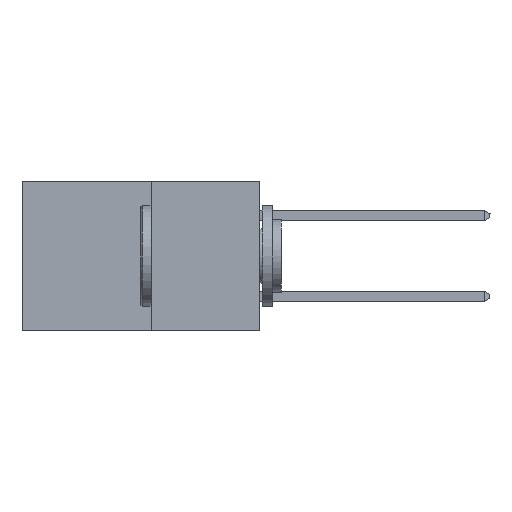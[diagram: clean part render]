
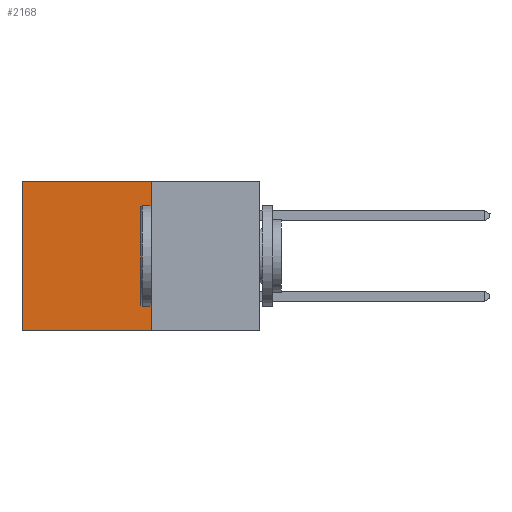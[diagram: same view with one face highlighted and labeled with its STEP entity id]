
A CAD part, left-side view. The second image highlights one B-rep face of the part: STEP entity #2168.
In plain terms, the highlighted planar face has unit normal (-1, 0, 0).
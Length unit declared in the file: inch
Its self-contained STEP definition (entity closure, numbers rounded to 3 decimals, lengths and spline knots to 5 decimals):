
#132 = CARTESIAN_POINT ( 'NONE',  ( 0.277, 0.27, -0.37 ) ) ;
#509 = ORIENTED_EDGE ( 'NONE', *, *, #4136, .F. ) ;
#1045 = AXIS2_PLACEMENT_3D ( 'NONE', #10286, #4081, #6554 ) ;
#1099 = VERTEX_POINT ( 'NONE', #3480 ) ;
#1236 = DIRECTION ( 'NONE',  ( 0., 1., 0. ) ) ;
#1237 = VECTOR ( 'NONE', #8139, 39.37008 ) ;
#1461 = PLANE ( 'NONE',  #1045 ) ;
#1806 = VERTEX_POINT ( 'NONE', #9484 ) ;
#2168 = ADVANCED_FACE ( 'NONE', ( #11413 ), #1461, .F. ) ;
#2413 = VECTOR ( 'NONE', #1236, 39.37008 ) ;
#2660 = ORIENTED_EDGE ( 'NONE', *, *, #3289, .T. ) ;
#2958 = ORIENTED_EDGE ( 'NONE', *, *, #7991, .T. ) ;
#3289 = EDGE_CURVE ( 'NONE', #1099, #1806, #9370, .T. ) ;
#3476 = CARTESIAN_POINT ( 'NONE',  ( 0.277, 0.27, 0. ) ) ;
#3480 = CARTESIAN_POINT ( 'NONE',  ( 0.277, 0.59, 0. ) ) ;
#3485 = EDGE_CURVE ( 'NONE', #10256, #1806, #10168, .T. ) ;
#4081 = DIRECTION ( 'NONE',  ( 1., 0., 0. ) ) ;
#4136 = EDGE_CURVE ( 'NONE', #8052, #10256, #4891, .T. ) ;
#4791 = DIRECTION ( 'NONE',  ( 0., 0., -1. ) ) ;
#4885 = CARTESIAN_POINT ( 'NONE',  ( 0.277, 0.27, -0.37 ) ) ;
#4891 = LINE ( 'NONE', #4885, #1237 ) ;
#4918 = EDGE_LOOP ( 'NONE', ( #2660, #5343, #509, #2958 ) ) ;
#5343 = ORIENTED_EDGE ( 'NONE', *, *, #3485, .F. ) ;
#6554 = DIRECTION ( 'NONE',  ( 0., 0., -1. ) ) ;
#7307 = DIRECTION ( 'NONE',  ( 0., 1., 0. ) ) ;
#7991 = EDGE_CURVE ( 'NONE', #8052, #1099, #11848, .T. ) ;
#8052 = VERTEX_POINT ( 'NONE', #3476 ) ;
#8139 = DIRECTION ( 'NONE',  ( 0., 0., -1. ) ) ;
#8252 = CARTESIAN_POINT ( 'NONE',  ( 0.277, 0.27, -0.37 ) ) ;
#9305 = VECTOR ( 'NONE', #7307, 39.37008 ) ;
#9370 = LINE ( 'NONE', #10661, #11386 ) ;
#9484 = CARTESIAN_POINT ( 'NONE',  ( 0.277, 0.59, -0.37 ) ) ;
#10040 = CARTESIAN_POINT ( 'NONE',  ( 0.277, 0.27, 0. ) ) ;
#10168 = LINE ( 'NONE', #132, #2413 ) ;
#10256 = VERTEX_POINT ( 'NONE', #8252 ) ;
#10286 = CARTESIAN_POINT ( 'NONE',  ( 0.277, 0.27, -0.37 ) ) ;
#10661 = CARTESIAN_POINT ( 'NONE',  ( 0.277, 0.59, -0.37 ) ) ;
#11386 = VECTOR ( 'NONE', #4791, 39.37008 ) ;
#11413 = FACE_OUTER_BOUND ( 'NONE', #4918, .T. ) ;
#11848 = LINE ( 'NONE', #10040, #9305 ) ;
